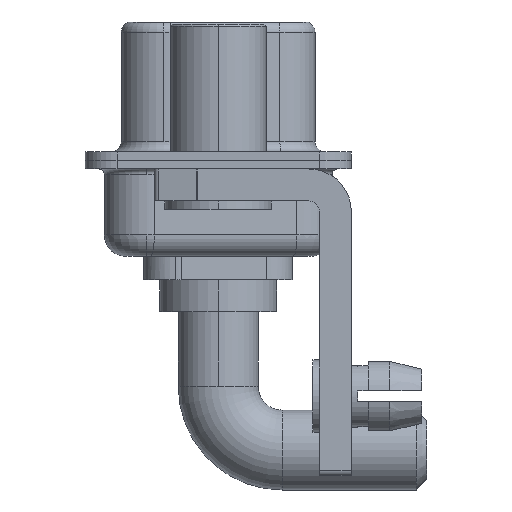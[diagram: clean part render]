
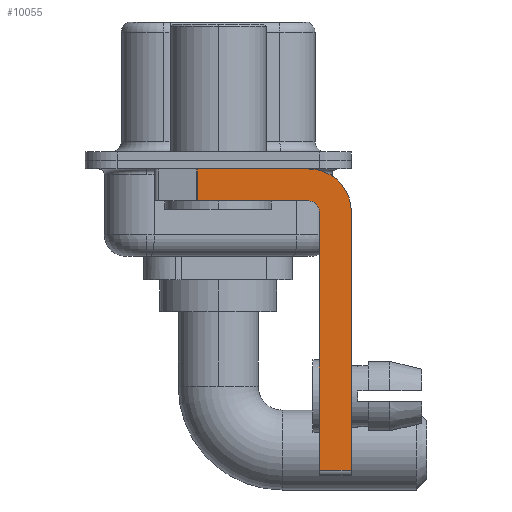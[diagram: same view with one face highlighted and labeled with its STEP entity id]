
A CAD part, left-side view. The second image highlights one B-rep face of the part: STEP entity #10055.
In plain terms, the highlighted planar face has unit normal (-1, 0, 0).
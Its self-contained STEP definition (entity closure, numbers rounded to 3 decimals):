
#237 = CARTESIAN_POINT ( 'NONE',  ( -2.9, 0.978, -1.9 ) ) ;
#250 = VERTEX_POINT ( 'NONE', #17415 ) ;
#445 = VERTEX_POINT ( 'NONE', #9516 ) ;
#720 = VECTOR ( 'NONE', #15516, 1000. ) ;
#1324 = DIRECTION ( 'NONE',  ( -1., 0., 0. ) ) ;
#1577 = DIRECTION ( 'NONE',  ( 1., 0., 0. ) ) ;
#1597 = DIRECTION ( 'NONE',  ( 0., 0., -1. ) ) ;
#1704 = AXIS2_PLACEMENT_3D ( 'NONE', #12029, #1324, #16314 ) ;
#1722 = AXIS2_PLACEMENT_3D ( 'NONE', #14061, #11416, #15609 ) ;
#2867 = CARTESIAN_POINT ( 'NONE',  ( -2.9, -4.75, -2.4 ) ) ;
#3096 = VERTEX_POINT ( 'NONE', #5593 ) ;
#3747 = VERTEX_POINT ( 'NONE', #12465 ) ;
#4448 = ORIENTED_EDGE ( 'NONE', *, *, #16766, .F. ) ;
#4505 = LINE ( 'NONE', #19207, #11413 ) ;
#4603 = FACE_OUTER_BOUND ( 'NONE', #11450, .T. ) ;
#5258 = ORIENTED_EDGE ( 'NONE', *, *, #15854, .F. ) ;
#5574 = CARTESIAN_POINT ( 'NONE',  ( -2.9, -4.25, -14.55 ) ) ;
#5593 = CARTESIAN_POINT ( 'NONE',  ( -2.9, -4.25, -0.4 ) ) ;
#5715 = ORIENTED_EDGE ( 'NONE', *, *, #14176, .T. ) ;
#6544 = ORIENTED_EDGE ( 'NONE', *, *, #16190, .F. ) ;
#6904 = VECTOR ( 'NONE', #1597, 1000. ) ;
#7512 = DIRECTION ( 'NONE',  ( 0., 0., -1. ) ) ;
#8005 = VERTEX_POINT ( 'NONE', #2867 ) ;
#8043 = EDGE_CURVE ( 'NONE', #445, #8641, #13214, .T. ) ;
#8228 = CIRCLE ( 'NONE', #1704, 0.5 ) ;
#8641 = VERTEX_POINT ( 'NONE', #237 ) ;
#9189 = ORIENTED_EDGE ( 'NONE', *, *, #8043, .T. ) ;
#9468 = CARTESIAN_POINT ( 'NONE',  ( -2.9, -4.75, -14.8 ) ) ;
#9516 = CARTESIAN_POINT ( 'NONE',  ( -2.9, 0.978, -0.4 ) ) ;
#9645 = CARTESIAN_POINT ( 'NONE',  ( -2.9, -6.25, -2.4 ) ) ;
#9814 = VECTOR ( 'NONE', #13429, 1000. ) ;
#10012 = EDGE_CURVE ( 'NONE', #445, #3096, #4505, .T. ) ;
#10055 = ADVANCED_FACE ( 'NONE', ( #4603 ), #17650, .F. ) ;
#10441 = CARTESIAN_POINT ( 'NONE',  ( -2.9, -4.25, -2.4 ) ) ;
#11259 = LINE ( 'NONE', #18654, #15104 ) ;
#11413 = VECTOR ( 'NONE', #11803, 1000. ) ;
#11416 = DIRECTION ( 'NONE',  ( 1., 0., 0. ) ) ;
#11450 = EDGE_LOOP ( 'NONE', ( #12037, #9189, #4448, #5258, #14789, #5715, #15109, #6544 ) ) ;
#11803 = DIRECTION ( 'NONE',  ( 0., -1., 0. ) ) ;
#12029 = CARTESIAN_POINT ( 'NONE',  ( -2.9, -4.25, -2.4 ) ) ;
#12037 = ORIENTED_EDGE ( 'NONE', *, *, #10012, .F. ) ;
#12465 = CARTESIAN_POINT ( 'NONE',  ( -2.9, -4.75, -14.55 ) ) ;
#13088 = LINE ( 'NONE', #5574, #18418 ) ;
#13214 = LINE ( 'NONE', #14872, #6904 ) ;
#13429 = DIRECTION ( 'NONE',  ( 0., 1., 0. ) ) ;
#13943 = EDGE_CURVE ( 'NONE', #3747, #8005, #14052, .T. ) ;
#14052 = LINE ( 'NONE', #9468, #720 ) ;
#14061 = CARTESIAN_POINT ( 'NONE',  ( -2.9, -4.25, -2.4 ) ) ;
#14110 = DIRECTION ( 'NONE',  ( 0., 0., -1. ) ) ;
#14176 = EDGE_CURVE ( 'NONE', #3747, #17348, #13088, .T. ) ;
#14350 = CARTESIAN_POINT ( 'NONE',  ( -2.9, -6.25, -14.55 ) ) ;
#14789 = ORIENTED_EDGE ( 'NONE', *, *, #13943, .F. ) ;
#14872 = CARTESIAN_POINT ( 'NONE',  ( -2.9, 0.978, -1.9 ) ) ;
#14896 = AXIS2_PLACEMENT_3D ( 'NONE', #10441, #1577, #7512 ) ;
#14987 = LINE ( 'NONE', #16339, #9814 ) ;
#15104 = VECTOR ( 'NONE', #14110, 1000. ) ;
#15109 = ORIENTED_EDGE ( 'NONE', *, *, #16356, .F. ) ;
#15516 = DIRECTION ( 'NONE',  ( 0., 0., 1. ) ) ;
#15609 = DIRECTION ( 'NONE',  ( 0., 0., -1. ) ) ;
#15854 = EDGE_CURVE ( 'NONE', #8005, #250, #8228, .T. ) ;
#16190 = EDGE_CURVE ( 'NONE', #3096, #17925, #18791, .T. ) ;
#16314 = DIRECTION ( 'NONE',  ( 0., 0., 1. ) ) ;
#16339 = CARTESIAN_POINT ( 'NONE',  ( -2.9, -4.25, -1.9 ) ) ;
#16356 = EDGE_CURVE ( 'NONE', #17925, #17348, #11259, .T. ) ;
#16766 = EDGE_CURVE ( 'NONE', #250, #8641, #14987, .T. ) ;
#17348 = VERTEX_POINT ( 'NONE', #14350 ) ;
#17415 = CARTESIAN_POINT ( 'NONE',  ( -2.9, -4.25, -1.9 ) ) ;
#17442 = DIRECTION ( 'NONE',  ( 0., -1., 0. ) ) ;
#17650 = PLANE ( 'NONE',  #14896 ) ;
#17925 = VERTEX_POINT ( 'NONE', #9645 ) ;
#18418 = VECTOR ( 'NONE', #17442, 1000. ) ;
#18654 = CARTESIAN_POINT ( 'NONE',  ( -2.9, -6.25, -2.4 ) ) ;
#18791 = CIRCLE ( 'NONE', #1722, 2. ) ;
#19207 = CARTESIAN_POINT ( 'NONE',  ( -2.9, 3., -0.4 ) ) ;
